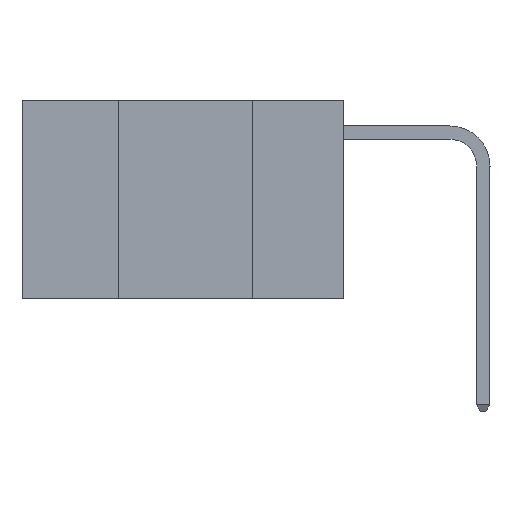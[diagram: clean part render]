
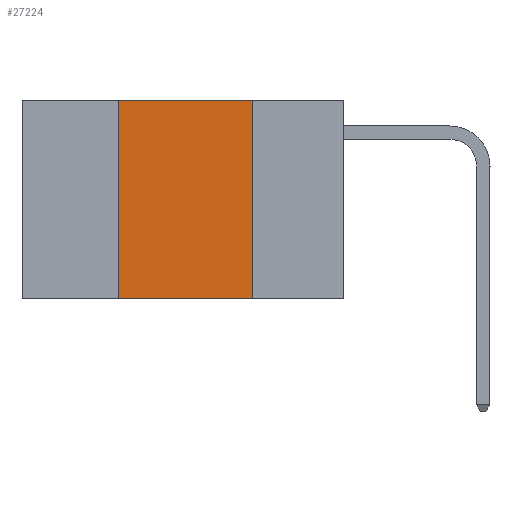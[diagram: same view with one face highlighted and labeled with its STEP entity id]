
A CAD part, left-side view. The second image highlights one B-rep face of the part: STEP entity #27224.
In plain terms, the highlighted planar face has unit normal (-1, 0, 0).
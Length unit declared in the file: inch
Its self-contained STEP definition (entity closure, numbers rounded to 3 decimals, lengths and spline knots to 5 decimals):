
#1688 = CARTESIAN_POINT ( 'NONE',  ( 0., 0.42, 0. ) ) ;
#1886 = ORIENTED_EDGE ( 'NONE', *, *, #25015, .F. ) ;
#2558 = DIRECTION ( 'NONE',  ( 1., 0., 0. ) ) ;
#2695 = VECTOR ( 'NONE', #14081, 39.37008 ) ;
#3012 = VERTEX_POINT ( 'NONE', #16375 ) ;
#3153 = CARTESIAN_POINT ( 'NONE',  ( 0., 0.6, 0. ) ) ;
#3563 = DIRECTION ( 'NONE',  ( 0., 0., -1. ) ) ;
#4565 = VECTOR ( 'NONE', #14623, 39.37008 ) ;
#4620 = CARTESIAN_POINT ( 'NONE',  ( 0., 0.17, 0. ) ) ;
#7674 = VERTEX_POINT ( 'NONE', #26114 ) ;
#8495 = ORIENTED_EDGE ( 'NONE', *, *, #14641, .F. ) ;
#8621 = LINE ( 'NONE', #3153, #2695 ) ;
#9121 = VECTOR ( 'NONE', #25285, 39.37008 ) ;
#9154 = PLANE ( 'NONE',  #14351 ) ;
#9168 = ORIENTED_EDGE ( 'NONE', *, *, #16603, .T. ) ;
#9784 = LINE ( 'NONE', #1688, #9121 ) ;
#10210 = CARTESIAN_POINT ( 'NONE',  ( 0., 0.17, 0. ) ) ;
#12831 = VERTEX_POINT ( 'NONE', #17155 ) ;
#13486 = CARTESIAN_POINT ( 'NONE',  ( 0., 0.6, 0. ) ) ;
#14081 = DIRECTION ( 'NONE',  ( 0., -1., 0. ) ) ;
#14351 = AXIS2_PLACEMENT_3D ( 'NONE', #13486, #2558, #17741 ) ;
#14578 = LINE ( 'NONE', #10210, #25035 ) ;
#14623 = DIRECTION ( 'NONE',  ( 0., -1., 0. ) ) ;
#14641 = EDGE_CURVE ( 'NONE', #7674, #3012, #9784, .T. ) ;
#16375 = CARTESIAN_POINT ( 'NONE',  ( 0., 0.42, 0. ) ) ;
#16603 = EDGE_CURVE ( 'NONE', #7674, #12831, #25220, .T. ) ;
#17155 = CARTESIAN_POINT ( 'NONE',  ( 0., 0.17, -0.37 ) ) ;
#17741 = DIRECTION ( 'NONE',  ( 0., 0., -1. ) ) ;
#18498 = ORIENTED_EDGE ( 'NONE', *, *, #26875, .F. ) ;
#23026 = CARTESIAN_POINT ( 'NONE',  ( 0., 0.6, -0.37 ) ) ;
#23349 = VERTEX_POINT ( 'NONE', #4620 ) ;
#25015 = EDGE_CURVE ( 'NONE', #3012, #23349, #8621, .T. ) ;
#25035 = VECTOR ( 'NONE', #3563, 39.37008 ) ;
#25220 = LINE ( 'NONE', #23026, #4565 ) ;
#25285 = DIRECTION ( 'NONE',  ( 0., 0., 1. ) ) ;
#26114 = CARTESIAN_POINT ( 'NONE',  ( 0., 0.42, -0.37 ) ) ;
#26592 = EDGE_LOOP ( 'NONE', ( #18498, #1886, #8495, #9168 ) ) ;
#26875 = EDGE_CURVE ( 'NONE', #23349, #12831, #14578, .T. ) ;
#26920 = FACE_OUTER_BOUND ( 'NONE', #26592, .T. ) ;
#27224 = ADVANCED_FACE ( 'NONE', ( #26920 ), #9154, .F. ) ;
